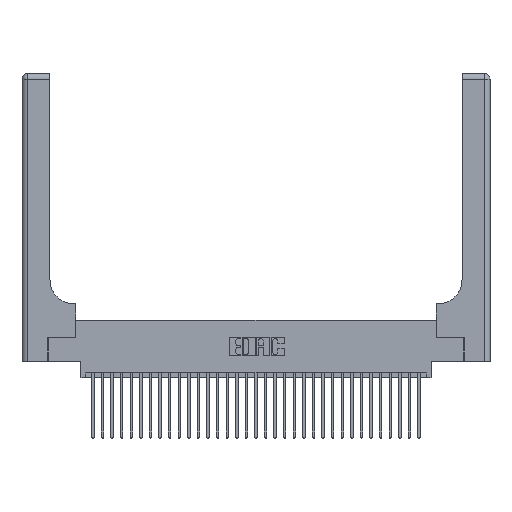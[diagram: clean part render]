
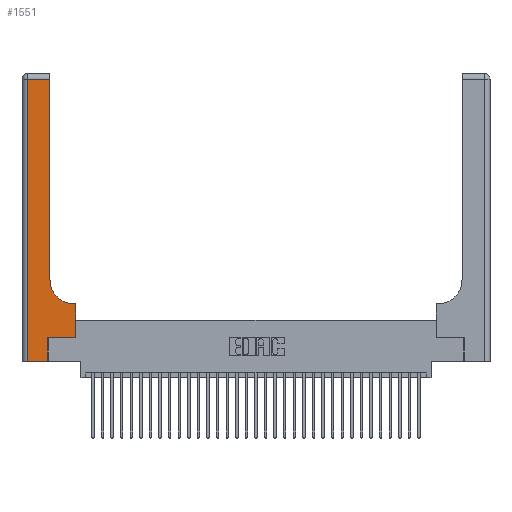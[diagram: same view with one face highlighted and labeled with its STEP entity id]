
A CAD part, top view. The second image highlights one B-rep face of the part: STEP entity #1551.
In plain terms, the highlighted planar face has unit normal (0, 0, 1).
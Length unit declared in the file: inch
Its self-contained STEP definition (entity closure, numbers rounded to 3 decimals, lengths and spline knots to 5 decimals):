
#496 = DIRECTION ( 'NONE',  ( 0., 0., -1. ) ) ;
#549 = ORIENTED_EDGE ( 'NONE', *, *, #16853, .T. ) ;
#709 = VECTOR ( 'NONE', #2223, 39.37008 ) ;
#1293 = LINE ( 'NONE', #1842, #24532 ) ;
#1551 = ADVANCED_FACE ( 'NONE', ( #14444 ), #22016, .F. ) ;
#1607 = CARTESIAN_POINT ( 'NONE',  ( 0.5585, 0.6, 0.37 ) ) ;
#1842 = CARTESIAN_POINT ( 'NONE',  ( 0., 0., 0.37 ) ) ;
#2223 = DIRECTION ( 'NONE',  ( 0., 1., 0. ) ) ;
#2270 = VERTEX_POINT ( 'NONE', #28982 ) ;
#2385 = VECTOR ( 'NONE', #11154, 39.37008 ) ;
#2514 = LINE ( 'NONE', #11908, #12694 ) ;
#5188 = LINE ( 'NONE', #17880, #709 ) ;
#5386 = LINE ( 'NONE', #12651, #6638 ) ;
#5459 = CARTESIAN_POINT ( 'NONE',  ( 0.06, 0., 0.37 ) ) ;
#6067 = EDGE_LOOP ( 'NONE', ( #13415, #31375, #18764, #6158, #10766, #23587, #14177, #549, #26049 ) ) ;
#6158 = ORIENTED_EDGE ( 'NONE', *, *, #17381, .T. ) ;
#6638 = VECTOR ( 'NONE', #8226, 39.37008 ) ;
#6677 = CARTESIAN_POINT ( 'NONE',  ( 0.06, 3., 0.37 ) ) ;
#6899 = VERTEX_POINT ( 'NONE', #5459 ) ;
#8226 = DIRECTION ( 'NONE',  ( -1., 0., 0. ) ) ;
#8785 = DIRECTION ( 'NONE',  ( 1., 0., 0. ) ) ;
#10087 = VERTEX_POINT ( 'NONE', #25302 ) ;
#10479 = EDGE_CURVE ( 'NONE', #11439, #10087, #28762, .T. ) ;
#10766 = ORIENTED_EDGE ( 'NONE', *, *, #33006, .T. ) ;
#10869 = DIRECTION ( 'NONE',  ( 1., 0., 0. ) ) ;
#10931 = LINE ( 'NONE', #13802, #2385 ) ;
#10968 = CARTESIAN_POINT ( 'NONE',  ( 0.269, 0.25, 0.37 ) ) ;
#11154 = DIRECTION ( 'NONE',  ( -1., 0., 0. ) ) ;
#11439 = VERTEX_POINT ( 'NONE', #14211 ) ;
#11535 = AXIS2_PLACEMENT_3D ( 'NONE', #12963, #496, #10869 ) ;
#11908 = CARTESIAN_POINT ( 'NONE',  ( 0.2915, 3., 0.37 ) ) ;
#11993 = CARTESIAN_POINT ( 'NONE',  ( 0.269, 0., 0.37 ) ) ;
#12651 = CARTESIAN_POINT ( 'NONE',  ( 0.2915, 0.6, 0.37 ) ) ;
#12694 = VECTOR ( 'NONE', #30256, 39.37008 ) ;
#12963 = CARTESIAN_POINT ( 'NONE',  ( 0.5415, 0.85, 0.37 ) ) ;
#13201 = EDGE_CURVE ( 'NONE', #16213, #19285, #5188, .T. ) ;
#13415 = ORIENTED_EDGE ( 'NONE', *, *, #17609, .T. ) ;
#13802 = CARTESIAN_POINT ( 'NONE',  ( 0., 2.94, 0.37 ) ) ;
#14003 = VERTEX_POINT ( 'NONE', #26411 ) ;
#14177 = ORIENTED_EDGE ( 'NONE', *, *, #13201, .T. ) ;
#14211 = CARTESIAN_POINT ( 'NONE',  ( 0.5415, 0.6, 0.37 ) ) ;
#14389 = DIRECTION ( 'NONE',  ( 0., 0., -1. ) ) ;
#14444 = FACE_OUTER_BOUND ( 'NONE', #6067, .T. ) ;
#14621 = DIRECTION ( 'NONE',  ( -1., 0., 0. ) ) ;
#14937 = VECTOR ( 'NONE', #32983, 39.37008 ) ;
#15370 = EDGE_CURVE ( 'NONE', #14003, #6899, #21840, .T. ) ;
#15867 = CARTESIAN_POINT ( 'NONE',  ( 0., 3., 0.37 ) ) ;
#16213 = VERTEX_POINT ( 'NONE', #23787 ) ;
#16737 = LINE ( 'NONE', #10968, #17565 ) ;
#16853 = EDGE_CURVE ( 'NONE', #19285, #11439, #5386, .T. ) ;
#17381 = EDGE_CURVE ( 'NONE', #6899, #32797, #1293, .T. ) ;
#17565 = VECTOR ( 'NONE', #8785, 39.37008 ) ;
#17609 = EDGE_CURVE ( 'NONE', #10087, #2270, #2514, .T. ) ;
#17880 = CARTESIAN_POINT ( 'NONE',  ( 0.5585, 0.25, 0.37 ) ) ;
#18764 = ORIENTED_EDGE ( 'NONE', *, *, #15370, .T. ) ;
#19285 = VERTEX_POINT ( 'NONE', #1607 ) ;
#21792 = VERTEX_POINT ( 'NONE', #22418 ) ;
#21840 = LINE ( 'NONE', #6677, #28379 ) ;
#22016 = PLANE ( 'NONE',  #32384 ) ;
#22418 = CARTESIAN_POINT ( 'NONE',  ( 0.269, 0.25, 0.37 ) ) ;
#22705 = DIRECTION ( 'NONE',  ( 1., 0., 0. ) ) ;
#22946 = CARTESIAN_POINT ( 'NONE',  ( 0.269, 0., 0.37 ) ) ;
#23587 = ORIENTED_EDGE ( 'NONE', *, *, #26433, .T. ) ;
#23787 = CARTESIAN_POINT ( 'NONE',  ( 0.5585, 0.25, 0.37 ) ) ;
#24532 = VECTOR ( 'NONE', #22705, 39.37008 ) ;
#25302 = CARTESIAN_POINT ( 'NONE',  ( 0.2915, 0.85, 0.37 ) ) ;
#26049 = ORIENTED_EDGE ( 'NONE', *, *, #10479, .T. ) ;
#26411 = CARTESIAN_POINT ( 'NONE',  ( 0.06, 2.94, 0.37 ) ) ;
#26433 = EDGE_CURVE ( 'NONE', #21792, #16213, #16737, .T. ) ;
#27113 = EDGE_CURVE ( 'NONE', #2270, #14003, #10931, .T. ) ;
#27131 = LINE ( 'NONE', #22946, #14937 ) ;
#28379 = VECTOR ( 'NONE', #32913, 39.37008 ) ;
#28762 = CIRCLE ( 'NONE', #11535, 0.25 ) ;
#28982 = CARTESIAN_POINT ( 'NONE',  ( 0.2915, 2.94, 0.37 ) ) ;
#30256 = DIRECTION ( 'NONE',  ( 0., 1., 0. ) ) ;
#31375 = ORIENTED_EDGE ( 'NONE', *, *, #27113, .T. ) ;
#32384 = AXIS2_PLACEMENT_3D ( 'NONE', #15867, #14389, #14621 ) ;
#32797 = VERTEX_POINT ( 'NONE', #11993 ) ;
#32913 = DIRECTION ( 'NONE',  ( 0., -1., 0. ) ) ;
#32983 = DIRECTION ( 'NONE',  ( 0., 1., 0. ) ) ;
#33006 = EDGE_CURVE ( 'NONE', #32797, #21792, #27131, .T. ) ;
